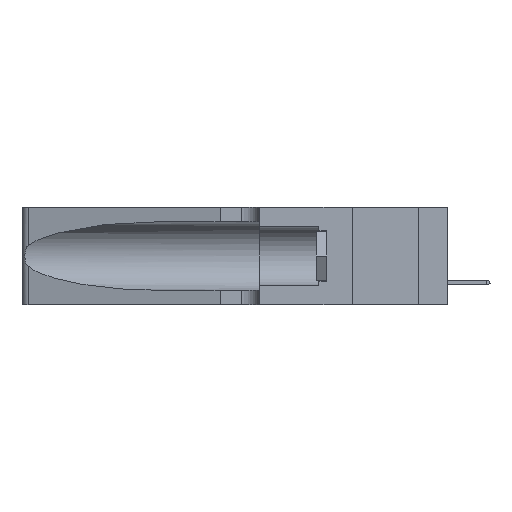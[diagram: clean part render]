
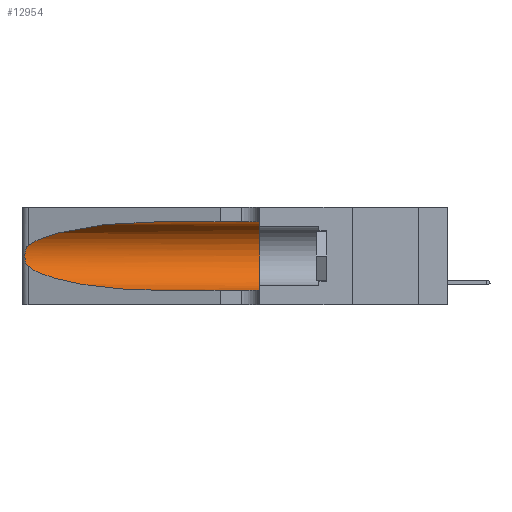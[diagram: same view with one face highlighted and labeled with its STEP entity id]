
A CAD part, left-side view. The second image highlights one B-rep face of the part: STEP entity #12954.
In plain terms, the highlighted cylindrical face has radius 3.308 mm (diameter 6.617 mm), a partial arc.
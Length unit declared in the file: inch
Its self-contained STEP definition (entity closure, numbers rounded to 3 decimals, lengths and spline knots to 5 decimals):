
#140 = CARTESIAN_POINT ( 'NONE',  ( 0.25854, 1.2359, 0.20912 ) ) ;
#524 = VERTEX_POINT ( 'NONE', #18980 ) ;
#682 = CARTESIAN_POINT ( 'NONE',  ( 0.1305, 1.61858, 0.05475 ) ) ;
#1541 = CARTESIAN_POINT ( 'NONE',  ( 0.25856, 1.23593, 0.16098 ) ) ;
#1640 = EDGE_LOOP ( 'NONE', ( #2428, #17911, #15197, #12175, #14451, #19766 ) ) ;
#1707 = CARTESIAN_POINT ( 'NONE',  ( 0.2373, 1.15595, 0.08982 ) ) ;
#1758 = CARTESIAN_POINT ( 'NONE',  ( 0.25487, 1.22718, 0.14631 ) ) ;
#2428 = ORIENTED_EDGE ( 'NONE', *, *, #4241, .T. ) ;
#2915 = DIRECTION ( 'NONE',  ( 0., -1., 0. ) ) ;
#2965 = AXIS2_PLACEMENT_3D ( 'NONE', #14627, #6721, #8319 ) ;
#3176 = VERTEX_POINT ( 'NONE', #12832 ) ;
#3371 = CARTESIAN_POINT ( 'NONE',  ( 0.25787, 1.23484, 0.2124 ) ) ;
#3634 = VERTEX_POINT ( 'NONE', #13573 ) ;
#3797 = B_SPLINE_CURVE_WITH_KNOTS ( 'NONE', 3,
 ( #18836, #12586, #16059, #3371, #140, #7885, #9395, #4912, #11015, #1541, #12847, #4777, #6550, #18902 ),
 .UNSPECIFIED., .F., .F.,
 ( 4, 2, 2, 2, 2, 2, 4 ),
 ( 0., 0.00027, 0.00053, 0.00107, 0.0016, 0.00187, 0.00214 ),
 .UNSPECIFIED. ) ;
#4241 = EDGE_CURVE ( 'NONE', #524, #18451, #5320, .T. ) ;
#4777 = CARTESIAN_POINT ( 'NONE',  ( 0.25639, 1.23186, 0.15144 ) ) ;
#4876 = CARTESIAN_POINT ( 'NONE',  ( 0.18966, 0.96281, 0.05475 ) ) ;
#4912 = CARTESIAN_POINT ( 'NONE',  ( 0.26075, 1.23896, 0.178 ) ) ;
#5204 = LINE ( 'NONE', #10881, #7935 ) ;
#5280 = CARTESIAN_POINT ( 'NONE',  ( 0.1305, 0.35, 0.05475 ) ) ;
#5320 =( BOUNDED_CURVE ( )  B_SPLINE_CURVE ( 3, ( #7277, #12306, #12101, #16890 ),
 .UNSPECIFIED., .F., .F. ) 
 B_SPLINE_CURVE_WITH_KNOTS ( ( 4, 4 ),
 ( 1.5708, 2.84003 ),
 .UNSPECIFIED. ) 
 CURVE ( )  GEOMETRIC_REPRESENTATION_ITEM ( )  RATIONAL_B_SPLINE_CURVE ( ( 1., 0.87, 0.87, 1. ) ) 
 REPRESENTATION_ITEM ( '' )  );
#5375 = DIRECTION ( 'NONE',  ( 0., -1., 0. ) ) ;
#5793 = VECTOR ( 'NONE', #5375, 39.37008 ) ;
#5990 = AXIS2_PLACEMENT_3D ( 'NONE', #7566, #17237, #15731 ) ;
#6550 = CARTESIAN_POINT ( 'NONE',  ( 0.25555, 1.22993, 0.14849 ) ) ;
#6675 = CIRCLE ( 'NONE', #2965, 0.13025 ) ;
#6721 = DIRECTION ( 'NONE',  ( 0., 1., 0. ) ) ;
#7277 = CARTESIAN_POINT ( 'NONE',  ( 0.1305, 0.72297, 0.31525 ) ) ;
#7566 = CARTESIAN_POINT ( 'NONE',  ( 0.1305, 1.61858, 0.185 ) ) ;
#7885 = CARTESIAN_POINT ( 'NONE',  ( 0.26018, 1.23835, 0.19895 ) ) ;
#7935 = VECTOR ( 'NONE', #2915, 39.37008 ) ;
#8312 = FACE_OUTER_BOUND ( 'NONE', #1640, .T. ) ;
#8319 = DIRECTION ( 'NONE',  ( 0., 0., 1. ) ) ;
#9395 = CARTESIAN_POINT ( 'NONE',  ( 0.26075, 1.23896, 0.19203 ) ) ;
#9761 = CARTESIAN_POINT ( 'NONE',  ( 0.25487, 1.22718, 0.22369 ) ) ;
#10782 = VERTEX_POINT ( 'NONE', #5280 ) ;
#10881 = CARTESIAN_POINT ( 'NONE',  ( 0.1305, 1.61858, 0.31525 ) ) ;
#11015 = CARTESIAN_POINT ( 'NONE',  ( 0.26017, 1.23833, 0.17102 ) ) ;
#11180 =( BOUNDED_CURVE ( )  B_SPLINE_CURVE ( 3, ( #16091, #1707, #4876, #15955 ),
 .UNSPECIFIED., .F., .T. ) 
 B_SPLINE_CURVE_WITH_KNOTS ( ( 4, 4 ),
 ( 3.44316, 4.71239 ),
 .UNSPECIFIED. ) 
 CURVE ( )  GEOMETRIC_REPRESENTATION_ITEM ( )  RATIONAL_B_SPLINE_CURVE ( ( 1., 0.87, 0.87, 1. ) ) 
 REPRESENTATION_ITEM ( '' )  );
#11761 = EDGE_CURVE ( 'NONE', #13053, #3176, #11180, .T. ) ;
#12101 = CARTESIAN_POINT ( 'NONE',  ( 0.2373, 1.15595, 0.28018 ) ) ;
#12175 = ORIENTED_EDGE ( 'NONE', *, *, #18824, .T. ) ;
#12306 = CARTESIAN_POINT ( 'NONE',  ( 0.18966, 0.96281, 0.31525 ) ) ;
#12586 = CARTESIAN_POINT ( 'NONE',  ( 0.25555, 1.22994, 0.2215 ) ) ;
#12832 = CARTESIAN_POINT ( 'NONE',  ( 0.1305, 0.72297, 0.05475 ) ) ;
#12847 = CARTESIAN_POINT ( 'NONE',  ( 0.25789, 1.23486, 0.15765 ) ) ;
#12954 = ADVANCED_FACE ( 'NONE', ( #8312 ), #18682, .F. ) ;
#13053 = VERTEX_POINT ( 'NONE', #1758 ) ;
#13573 = CARTESIAN_POINT ( 'NONE',  ( 0.1305, 0.35, 0.31525 ) ) ;
#14451 = ORIENTED_EDGE ( 'NONE', *, *, #14980, .F. ) ;
#14469 = LINE ( 'NONE', #682, #5793 ) ;
#14627 = CARTESIAN_POINT ( 'NONE',  ( 0.1305, 0.35, 0.185 ) ) ;
#14852 = EDGE_CURVE ( 'NONE', #524, #3634, #5204, .T. ) ;
#14980 = EDGE_CURVE ( 'NONE', #3634, #10782, #6675, .T. ) ;
#15197 = ORIENTED_EDGE ( 'NONE', *, *, #11761, .T. ) ;
#15731 = DIRECTION ( 'NONE',  ( 0., 0., -1. ) ) ;
#15955 = CARTESIAN_POINT ( 'NONE',  ( 0.1305, 0.72297, 0.05475 ) ) ;
#16059 = CARTESIAN_POINT ( 'NONE',  ( 0.25639, 1.23184, 0.21858 ) ) ;
#16091 = CARTESIAN_POINT ( 'NONE',  ( 0.25487, 1.22718, 0.14631 ) ) ;
#16890 = CARTESIAN_POINT ( 'NONE',  ( 0.25487, 1.22718, 0.22369 ) ) ;
#17237 = DIRECTION ( 'NONE',  ( 0., -1., 0. ) ) ;
#17738 = EDGE_CURVE ( 'NONE', #18451, #13053, #3797, .T. ) ;
#17911 = ORIENTED_EDGE ( 'NONE', *, *, #17738, .T. ) ;
#18451 = VERTEX_POINT ( 'NONE', #9761 ) ;
#18682 = CYLINDRICAL_SURFACE ( 'NONE', #5990, 0.13025 ) ;
#18824 = EDGE_CURVE ( 'NONE', #3176, #10782, #14469, .T. ) ;
#18836 = CARTESIAN_POINT ( 'NONE',  ( 0.25487, 1.22718, 0.22369 ) ) ;
#18902 = CARTESIAN_POINT ( 'NONE',  ( 0.25487, 1.22718, 0.14631 ) ) ;
#18980 = CARTESIAN_POINT ( 'NONE',  ( 0.1305, 0.72297, 0.31525 ) ) ;
#19766 = ORIENTED_EDGE ( 'NONE', *, *, #14852, .F. ) ;
